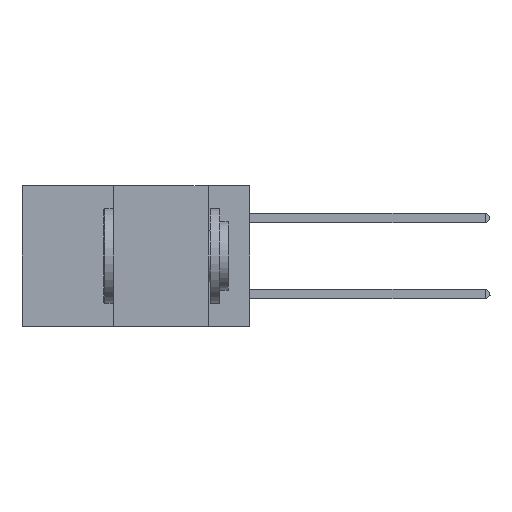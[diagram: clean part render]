
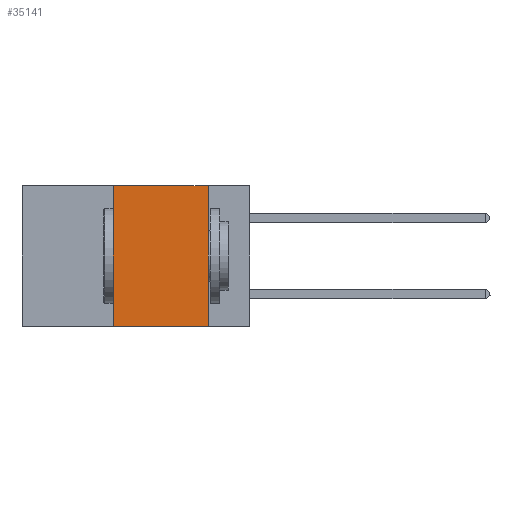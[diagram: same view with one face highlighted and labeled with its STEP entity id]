
A CAD part, left-side view. The second image highlights one B-rep face of the part: STEP entity #35141.
In plain terms, the highlighted planar face has unit normal (-1, 0, 0).
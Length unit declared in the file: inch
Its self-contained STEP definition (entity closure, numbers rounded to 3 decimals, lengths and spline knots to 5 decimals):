
#174 = DIRECTION ( 'NONE',  ( 0., -1., 0. ) ) ;
#1019 = CARTESIAN_POINT ( 'NONE',  ( 0., 0.36, -0.37 ) ) ;
#4318 = LINE ( 'NONE', #6959, #8120 ) ;
#4864 = CARTESIAN_POINT ( 'NONE',  ( 0., 0.11, -0.37 ) ) ;
#6567 = CARTESIAN_POINT ( 'NONE',  ( 0., 0.6, 0. ) ) ;
#6826 = ORIENTED_EDGE ( 'NONE', *, *, #24372, .F. ) ;
#6842 = VECTOR ( 'NONE', #41161, 39.37008 ) ;
#6959 = CARTESIAN_POINT ( 'NONE',  ( 0., 0.6, 0. ) ) ;
#7037 = DIRECTION ( 'NONE',  ( 0., 0., -1. ) ) ;
#7072 = LINE ( 'NONE', #18798, #9772 ) ;
#8120 = VECTOR ( 'NONE', #174, 39.37008 ) ;
#8800 = EDGE_CURVE ( 'NONE', #26706, #44495, #7072, .T. ) ;
#9207 = EDGE_CURVE ( 'NONE', #37946, #35323, #4318, .T. ) ;
#9772 = VECTOR ( 'NONE', #25942, 39.37008 ) ;
#10813 = CARTESIAN_POINT ( 'NONE',  ( 0., 0.11, 0. ) ) ;
#11592 = EDGE_CURVE ( 'NONE', #26706, #37946, #13990, .T. ) ;
#12417 = ORIENTED_EDGE ( 'NONE', *, *, #9207, .F. ) ;
#13990 = LINE ( 'NONE', #34128, #6842 ) ;
#15051 = AXIS2_PLACEMENT_3D ( 'NONE', #6567, #31725, #7037 ) ;
#18798 = CARTESIAN_POINT ( 'NONE',  ( 0., 0.6, -0.37 ) ) ;
#18936 = LINE ( 'NONE', #10813, #39269 ) ;
#19582 = FACE_OUTER_BOUND ( 'NONE', #23215, .T. ) ;
#21123 = PLANE ( 'NONE',  #15051 ) ;
#23215 = EDGE_LOOP ( 'NONE', ( #6826, #12417, #39617, #36453 ) ) ;
#24372 = EDGE_CURVE ( 'NONE', #35323, #44495, #18936, .T. ) ;
#25942 = DIRECTION ( 'NONE',  ( 0., -1., 0. ) ) ;
#26706 = VERTEX_POINT ( 'NONE', #1019 ) ;
#31725 = DIRECTION ( 'NONE',  ( 1., 0., 0. ) ) ;
#31985 = DIRECTION ( 'NONE',  ( 0., 0., -1. ) ) ;
#34126 = CARTESIAN_POINT ( 'NONE',  ( 0., 0.36, 0. ) ) ;
#34128 = CARTESIAN_POINT ( 'NONE',  ( 0., 0.36, 0. ) ) ;
#35141 = ADVANCED_FACE ( 'NONE', ( #19582 ), #21123, .F. ) ;
#35323 = VERTEX_POINT ( 'NONE', #42771 ) ;
#36453 = ORIENTED_EDGE ( 'NONE', *, *, #8800, .T. ) ;
#37946 = VERTEX_POINT ( 'NONE', #34126 ) ;
#39269 = VECTOR ( 'NONE', #31985, 39.37008 ) ;
#39617 = ORIENTED_EDGE ( 'NONE', *, *, #11592, .F. ) ;
#41161 = DIRECTION ( 'NONE',  ( 0., 0., 1. ) ) ;
#42771 = CARTESIAN_POINT ( 'NONE',  ( 0., 0.11, 0. ) ) ;
#44495 = VERTEX_POINT ( 'NONE', #4864 ) ;
